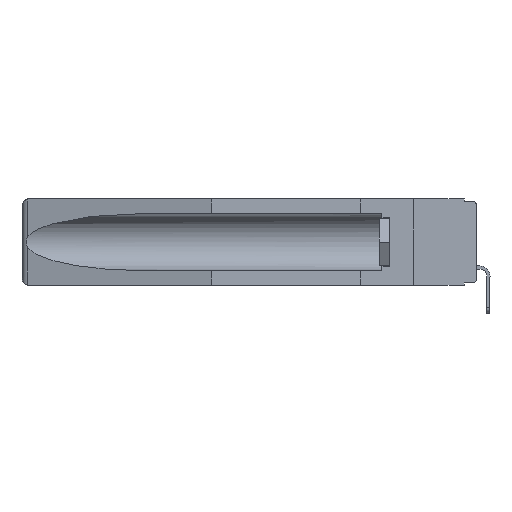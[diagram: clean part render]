
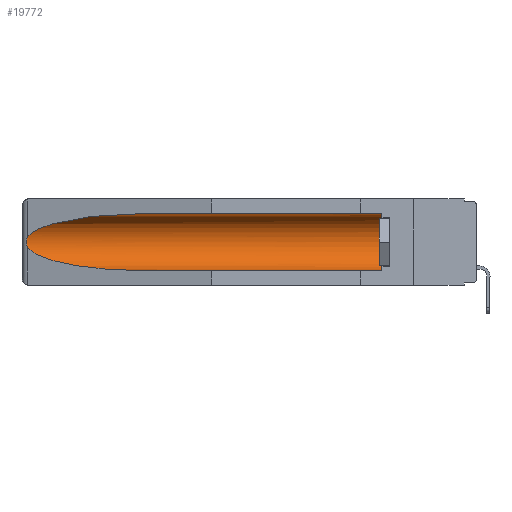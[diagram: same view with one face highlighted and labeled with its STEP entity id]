
A CAD part, left-side view. The second image highlights one B-rep face of the part: STEP entity #19772.
In plain terms, the highlighted cylindrical face has radius 2.857 mm (diameter 5.715 mm), a partial arc.
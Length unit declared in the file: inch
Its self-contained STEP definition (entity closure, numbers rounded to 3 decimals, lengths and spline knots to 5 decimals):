
#223 = CARTESIAN_POINT ( 'NONE',  ( 0.155, -0.30754, -0.059 ) ) ;
#473 = CARTESIAN_POINT ( 'NONE',  ( 0.26537, 1.52718, -0.14972 ) ) ;
#756 = ORIENTED_EDGE ( 'NONE', *, *, #10339, .T. ) ;
#793 = FACE_OUTER_BOUND ( 'NONE', #3716, .T. ) ;
#1703 = ORIENTED_EDGE ( 'NONE', *, *, #8241, .F. ) ;
#1813 = CARTESIAN_POINT ( 'NONE',  ( 0.155, -0.30754, -0.1715 ) ) ;
#2223 = CARTESIAN_POINT ( 'NONE',  ( 0.26654, 1.53092, -0.15636 ) ) ;
#2252 =( BOUNDED_CURVE ( )  B_SPLINE_CURVE ( 3, ( #7502, #15979, #16259, #18010 ),
 .UNSPECIFIED., .F., .F. ) 
 B_SPLINE_CURVE_WITH_KNOTS ( ( 4, 4 ),
 ( 0.1948, 1.5708 ),
 .UNSPECIFIED. ) 
 CURVE ( )  GEOMETRIC_REPRESENTATION_ITEM ( )  RATIONAL_B_SPLINE_CURVE ( ( 1., 0.848, 0.848, 1. ) ) 
 REPRESENTATION_ITEM ( '' )  );
#2429 = CARTESIAN_POINT ( 'NONE',  ( 0.155, 1.07973, -0.059 ) ) ;
#2660 = DIRECTION ( 'NONE',  ( 0., 1., 0. ) ) ;
#2897 = VECTOR ( 'NONE', #5247, 39.37008 ) ;
#2985 = CARTESIAN_POINT ( 'NONE',  ( 0.155, 1.07973, -0.059 ) ) ;
#3392 = CARTESIAN_POINT ( 'NONE',  ( 0.155, 1.07973, -0.284 ) ) ;
#3716 = EDGE_LOOP ( 'NONE', ( #10596, #756, #5581, #1703, #19300, #7550 ) ) ;
#4125 = CARTESIAN_POINT ( 'NONE',  ( 0.2673, 1.53269, -0.17917 ) ) ;
#4126 = AXIS2_PLACEMENT_3D ( 'NONE', #1813, #18742, #22314 ) ;
#4474 = CARTESIAN_POINT ( 'NONE',  ( 0.155, 0.126, -0.059 ) ) ;
#5247 = DIRECTION ( 'NONE',  ( 0., 1., 0. ) ) ;
#5460 = EDGE_CURVE ( 'NONE', #11215, #18916, #18058, .T. ) ;
#5581 = ORIENTED_EDGE ( 'NONE', *, *, #21436, .T. ) ;
#6510 = VERTEX_POINT ( 'NONE', #12742 ) ;
#7120 = CIRCLE ( 'NONE', #13137, 0.1125 ) ;
#7435 = VERTEX_POINT ( 'NONE', #3392 ) ;
#7502 = CARTESIAN_POINT ( 'NONE',  ( 0.26537, 1.52718, -0.19328 ) ) ;
#7550 = ORIENTED_EDGE ( 'NONE', *, *, #21185, .T. ) ;
#7660 = CARTESIAN_POINT ( 'NONE',  ( 0.155, -0.30754, -0.284 ) ) ;
#8012 = LINE ( 'NONE', #7660, #8283 ) ;
#8241 = EDGE_CURVE ( 'NONE', #12771, #7435, #8012, .T. ) ;
#8283 = VECTOR ( 'NONE', #2660, 39.37008 ) ;
#8856 = CARTESIAN_POINT ( 'NONE',  ( 0.155, 0.126, -0.1715 ) ) ;
#9248 = CARTESIAN_POINT ( 'NONE',  ( 0.2675, 1.53308, -0.16763 ) ) ;
#9334 = CARTESIAN_POINT ( 'NONE',  ( 0.26537, 1.52718, -0.19328 ) ) ;
#10339 = EDGE_CURVE ( 'NONE', #18916, #6510, #16684, .T. ) ;
#10596 = ORIENTED_EDGE ( 'NONE', *, *, #5460, .T. ) ;
#10621 = DIRECTION ( 'NONE',  ( 0., 0., 1. ) ) ;
#10832 = CYLINDRICAL_SURFACE ( 'NONE', #4126, 0.1125 ) ;
#11215 = VERTEX_POINT ( 'NONE', #2985 ) ;
#11259 = CARTESIAN_POINT ( 'NONE',  ( 0.155, 0.126, -0.284 ) ) ;
#12133 = EDGE_CURVE ( 'NONE', #12771, #20267, #7120, .T. ) ;
#12198 = DIRECTION ( 'NONE',  ( 0., -1., 0. ) ) ;
#12587 = CARTESIAN_POINT ( 'NONE',  ( 0.26597, 1.52961, -0.15275 ) ) ;
#12742 = CARTESIAN_POINT ( 'NONE',  ( 0.26537, 1.52718, -0.19328 ) ) ;
#12771 = VERTEX_POINT ( 'NONE', #11259 ) ;
#13090 = CARTESIAN_POINT ( 'NONE',  ( 0.26537, 1.52718, -0.14972 ) ) ;
#13137 = AXIS2_PLACEMENT_3D ( 'NONE', #8856, #12198, #10621 ) ;
#14477 = CARTESIAN_POINT ( 'NONE',  ( 0.2675, 1.53308, -0.17534 ) ) ;
#14531 = CARTESIAN_POINT ( 'NONE',  ( 0.25451, 1.48313, -0.09465 ) ) ;
#15979 = CARTESIAN_POINT ( 'NONE',  ( 0.25451, 1.48313, -0.24835 ) ) ;
#16148 = LINE ( 'NONE', #223, #2897 ) ;
#16259 = CARTESIAN_POINT ( 'NONE',  ( 0.21114, 1.30732, -0.284 ) ) ;
#16285 = CARTESIAN_POINT ( 'NONE',  ( 0.2673, 1.5327, -0.16383 ) ) ;
#16684 = B_SPLINE_CURVE_WITH_KNOTS ( 'NONE', 3,
 ( #473, #12587, #2223, #16285, #9248, #14477, #4125, #17959, #19701, #9334 ),
 .UNSPECIFIED., .F., .F.,
 ( 4, 2, 2, 2, 4 ),
 ( 0., 0.00029, 0.00058, 0.00087, 0.00117 ),
 .UNSPECIFIED. ) ;
#17959 = CARTESIAN_POINT ( 'NONE',  ( 0.26655, 1.53094, -0.18657 ) ) ;
#18010 = CARTESIAN_POINT ( 'NONE',  ( 0.155, 1.07973, -0.284 ) ) ;
#18058 =( BOUNDED_CURVE ( )  B_SPLINE_CURVE ( 3, ( #2429, #19824, #14531, #13090 ),
 .UNSPECIFIED., .F., .F. ) 
 B_SPLINE_CURVE_WITH_KNOTS ( ( 4, 4 ),
 ( 4.71239, 6.08839 ),
 .UNSPECIFIED. ) 
 CURVE ( )  GEOMETRIC_REPRESENTATION_ITEM ( )  RATIONAL_B_SPLINE_CURVE ( ( 1., 0.848, 0.848, 1. ) ) 
 REPRESENTATION_ITEM ( '' )  );
#18742 = DIRECTION ( 'NONE',  ( 0., 1., 0. ) ) ;
#18916 = VERTEX_POINT ( 'NONE', #21654 ) ;
#19300 = ORIENTED_EDGE ( 'NONE', *, *, #12133, .T. ) ;
#19701 = CARTESIAN_POINT ( 'NONE',  ( 0.26597, 1.5296, -0.19026 ) ) ;
#19772 = ADVANCED_FACE ( 'NONE', ( #793 ), #10832, .F. ) ;
#19824 = CARTESIAN_POINT ( 'NONE',  ( 0.21114, 1.30732, -0.059 ) ) ;
#20267 = VERTEX_POINT ( 'NONE', #4474 ) ;
#21185 = EDGE_CURVE ( 'NONE', #20267, #11215, #16148, .T. ) ;
#21436 = EDGE_CURVE ( 'NONE', #6510, #7435, #2252, .T. ) ;
#21654 = CARTESIAN_POINT ( 'NONE',  ( 0.26537, 1.52718, -0.14972 ) ) ;
#22314 = DIRECTION ( 'NONE',  ( 0., 0., 1. ) ) ;
